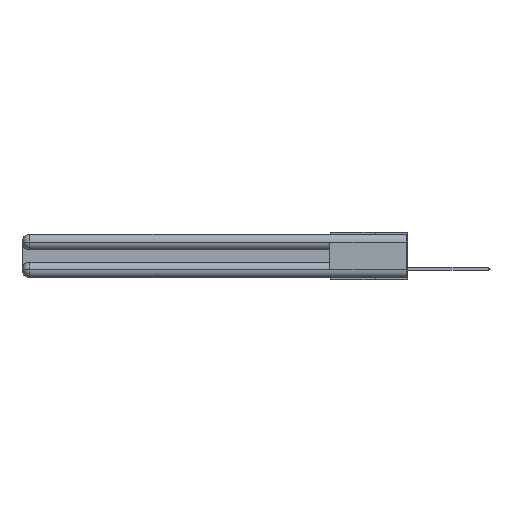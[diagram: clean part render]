
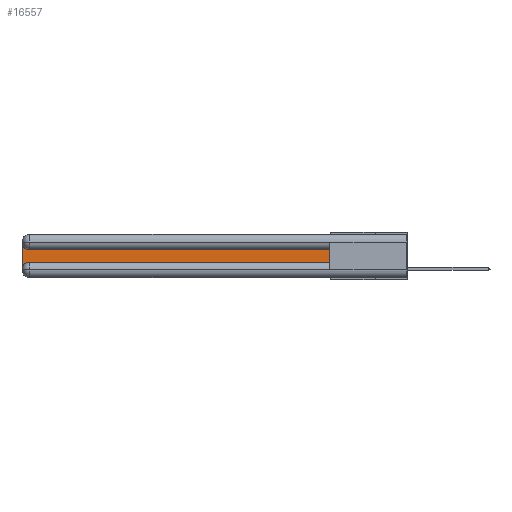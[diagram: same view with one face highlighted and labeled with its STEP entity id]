
A CAD part, left-side view. The second image highlights one B-rep face of the part: STEP entity #16557.
In plain terms, the highlighted planar face has unit normal (-1, 0, 0).
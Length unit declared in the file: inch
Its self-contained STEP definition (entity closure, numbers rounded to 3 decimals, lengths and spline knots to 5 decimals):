
#470 = LINE ( 'NONE', #9234, #7251 ) ;
#605 = EDGE_CURVE ( 'NONE', #18311, #9192, #19730, .T. ) ;
#793 = DIRECTION ( 'NONE',  ( 1., 0., 0. ) ) ;
#935 = ORIENTED_EDGE ( 'NONE', *, *, #14690, .T. ) ;
#1080 = ORIENTED_EDGE ( 'NONE', *, *, #28201, .T. ) ;
#1109 = CARTESIAN_POINT ( 'NONE',  ( 0.075, 0.6, -0.2175 ) ) ;
#1971 = DIRECTION ( 'NONE',  ( 0., 0., 1. ) ) ;
#5237 = VERTEX_POINT ( 'NONE', #17196 ) ;
#5897 = CARTESIAN_POINT ( 'NONE',  ( 0.075, 3., -0.2775 ) ) ;
#7251 = VECTOR ( 'NONE', #1971, 39.37008 ) ;
#7318 = AXIS2_PLACEMENT_3D ( 'NONE', #14318, #9141, #32167 ) ;
#7500 = ORIENTED_EDGE ( 'NONE', *, *, #21281, .T. ) ;
#9141 = DIRECTION ( 'NONE',  ( 1., 0., 0. ) ) ;
#9192 = VERTEX_POINT ( 'NONE', #5897 ) ;
#9234 = CARTESIAN_POINT ( 'NONE',  ( 0.075, 0.6, -0.2175 ) ) ;
#10572 = EDGE_CURVE ( 'NONE', #5237, #18311, #16968, .T. ) ;
#11284 = PLANE ( 'NONE',  #28032 ) ;
#11603 = DIRECTION ( 'NONE',  ( 0., -1., 0. ) ) ;
#12012 = CARTESIAN_POINT ( 'NONE',  ( 0.075, 0.6, -0.2175 ) ) ;
#12167 = DIRECTION ( 'NONE',  ( 0., 0., -1. ) ) ;
#12913 = VECTOR ( 'NONE', #12167, 39.37008 ) ;
#12954 = ORIENTED_EDGE ( 'NONE', *, *, #10572, .T. ) ;
#13650 = CARTESIAN_POINT ( 'NONE',  ( 0.075, 3., -0.1225 ) ) ;
#14223 = EDGE_CURVE ( 'NONE', #14293, #5237, #16874, .T. ) ;
#14293 = VERTEX_POINT ( 'NONE', #31256 ) ;
#14318 = CARTESIAN_POINT ( 'NONE',  ( 0.075, 2.94, -0.0625 ) ) ;
#14690 = EDGE_CURVE ( 'NONE', #9192, #17315, #27294, .T. ) ;
#15460 = CARTESIAN_POINT ( 'NONE',  ( 0.075, 0.6, -0.1225 ) ) ;
#16557 = ADVANCED_FACE ( 'NONE', ( #18337 ), #11284, .F. ) ;
#16874 = LINE ( 'NONE', #15460, #31724 ) ;
#16968 = CIRCLE ( 'NONE', #7318, 0.06 ) ;
#17196 = CARTESIAN_POINT ( 'NONE',  ( 0.075, 2.94, -0.1225 ) ) ;
#17315 = VERTEX_POINT ( 'NONE', #31425 ) ;
#18311 = VERTEX_POINT ( 'NONE', #32566 ) ;
#18337 = FACE_OUTER_BOUND ( 'NONE', #30922, .T. ) ;
#19321 = VERTEX_POINT ( 'NONE', #12012 ) ;
#19730 = LINE ( 'NONE', #27774, #12913 ) ;
#20493 = DIRECTION ( 'NONE',  ( 0., 1., 0. ) ) ;
#20526 = ORIENTED_EDGE ( 'NONE', *, *, #605, .T. ) ;
#21281 = EDGE_CURVE ( 'NONE', #19321, #14293, #470, .T. ) ;
#22180 = AXIS2_PLACEMENT_3D ( 'NONE', #25370, #30676, #27619 ) ;
#25370 = CARTESIAN_POINT ( 'NONE',  ( 0.075, 2.94, -0.2775 ) ) ;
#26589 = LINE ( 'NONE', #1109, #31048 ) ;
#26747 = DIRECTION ( 'NONE',  ( 0., 0., -1. ) ) ;
#27294 = CIRCLE ( 'NONE', #22180, 0.06 ) ;
#27619 = DIRECTION ( 'NONE',  ( 0., 0., -1. ) ) ;
#27774 = CARTESIAN_POINT ( 'NONE',  ( 0.075, 3., -0.2175 ) ) ;
#28032 = AXIS2_PLACEMENT_3D ( 'NONE', #13650, #793, #26747 ) ;
#28201 = EDGE_CURVE ( 'NONE', #17315, #19321, #26589, .T. ) ;
#30676 = DIRECTION ( 'NONE',  ( 1., 0., 0. ) ) ;
#30754 = ORIENTED_EDGE ( 'NONE', *, *, #14223, .T. ) ;
#30922 = EDGE_LOOP ( 'NONE', ( #30754, #12954, #20526, #935, #1080, #7500 ) ) ;
#31048 = VECTOR ( 'NONE', #11603, 39.37008 ) ;
#31256 = CARTESIAN_POINT ( 'NONE',  ( 0.075, 0.6, -0.1225 ) ) ;
#31425 = CARTESIAN_POINT ( 'NONE',  ( 0.075, 2.94, -0.2175 ) ) ;
#31724 = VECTOR ( 'NONE', #20493, 39.37008 ) ;
#32167 = DIRECTION ( 'NONE',  ( 0., 0., -1. ) ) ;
#32566 = CARTESIAN_POINT ( 'NONE',  ( 0.075, 3., -0.0625 ) ) ;
